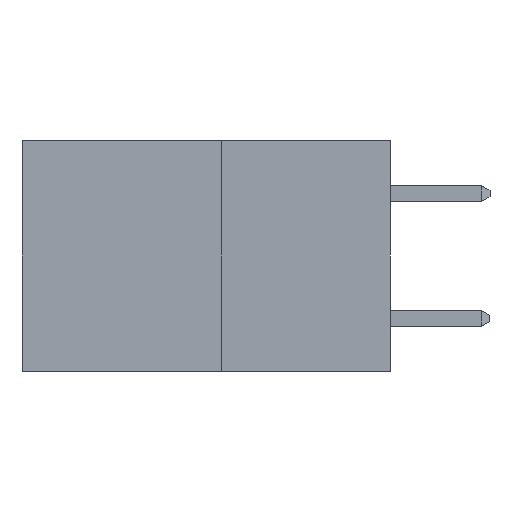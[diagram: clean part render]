
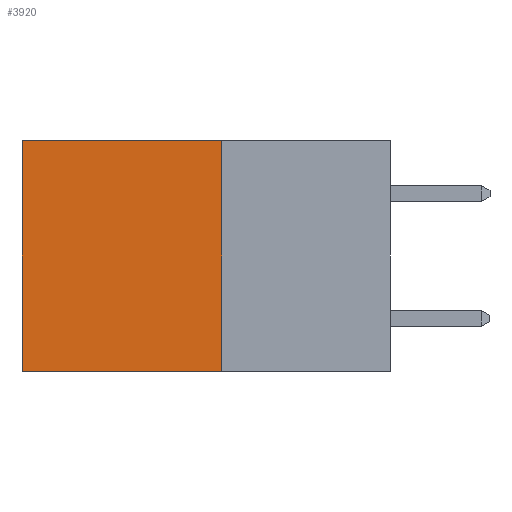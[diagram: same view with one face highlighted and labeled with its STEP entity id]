
A CAD part, left-side view. The second image highlights one B-rep face of the part: STEP entity #3920.
In plain terms, the highlighted planar face has unit normal (-1, 0, 0).
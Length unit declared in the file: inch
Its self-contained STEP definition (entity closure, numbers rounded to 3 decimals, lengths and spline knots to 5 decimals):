
#183 = EDGE_CURVE ( 'NONE', #2182, #4379, #7508, .T. ) ;
#225 = EDGE_CURVE ( 'NONE', #2569, #6240, #531, .T. ) ;
#531 = LINE ( 'NONE', #5180, #6972 ) ;
#741 = VECTOR ( 'NONE', #7719, 39.37008 ) ;
#815 = CARTESIAN_POINT ( 'NONE',  ( 0.277, 0.27, -0.37 ) ) ;
#1152 = DIRECTION ( 'NONE',  ( 1., 0., 0. ) ) ;
#1180 = LINE ( 'NONE', #7333, #4437 ) ;
#1643 = CARTESIAN_POINT ( 'NONE',  ( 0.277, 0.27, 0. ) ) ;
#1915 = LINE ( 'NONE', #815, #6741 ) ;
#2014 = CARTESIAN_POINT ( 'NONE',  ( 0.277, 0.27, -0.37 ) ) ;
#2048 = ORIENTED_EDGE ( 'NONE', *, *, #225, .F. ) ;
#2060 = DIRECTION ( 'NONE',  ( 0., 0., -1. ) ) ;
#2182 = VERTEX_POINT ( 'NONE', #4916 ) ;
#2569 = VERTEX_POINT ( 'NONE', #1643 ) ;
#3016 = DIRECTION ( 'NONE',  ( 0., 1., 0. ) ) ;
#3170 = CARTESIAN_POINT ( 'NONE',  ( 0.277, 0.59, -0.37 ) ) ;
#3315 = EDGE_CURVE ( 'NONE', #6240, #4379, #1915, .T. ) ;
#3332 = EDGE_LOOP ( 'NONE', ( #7292, #5657, #2048, #4216 ) ) ;
#3920 = ADVANCED_FACE ( 'NONE', ( #6645 ), #4804, .F. ) ;
#4216 = ORIENTED_EDGE ( 'NONE', *, *, #7146, .T. ) ;
#4226 = CARTESIAN_POINT ( 'NONE',  ( 0.277, 0.59, -0.37 ) ) ;
#4379 = VERTEX_POINT ( 'NONE', #3170 ) ;
#4437 = VECTOR ( 'NONE', #3016, 39.37008 ) ;
#4804 = PLANE ( 'NONE',  #6646 ) ;
#4916 = CARTESIAN_POINT ( 'NONE',  ( 0.277, 0.59, 0. ) ) ;
#5155 = DIRECTION ( 'NONE',  ( 0., 0., -1. ) ) ;
#5180 = CARTESIAN_POINT ( 'NONE',  ( 0.277, 0.27, -0.37 ) ) ;
#5657 = ORIENTED_EDGE ( 'NONE', *, *, #3315, .F. ) ;
#6124 = CARTESIAN_POINT ( 'NONE',  ( 0.277, 0.27, -0.37 ) ) ;
#6240 = VERTEX_POINT ( 'NONE', #6124 ) ;
#6645 = FACE_OUTER_BOUND ( 'NONE', #3332, .T. ) ;
#6646 = AXIS2_PLACEMENT_3D ( 'NONE', #2014, #1152, #2060 ) ;
#6741 = VECTOR ( 'NONE', #7494, 39.37008 ) ;
#6972 = VECTOR ( 'NONE', #5155, 39.37008 ) ;
#7146 = EDGE_CURVE ( 'NONE', #2569, #2182, #1180, .T. ) ;
#7292 = ORIENTED_EDGE ( 'NONE', *, *, #183, .T. ) ;
#7333 = CARTESIAN_POINT ( 'NONE',  ( 0.277, 0.27, 0. ) ) ;
#7494 = DIRECTION ( 'NONE',  ( 0., 1., 0. ) ) ;
#7508 = LINE ( 'NONE', #4226, #741 ) ;
#7719 = DIRECTION ( 'NONE',  ( 0., 0., -1. ) ) ;
